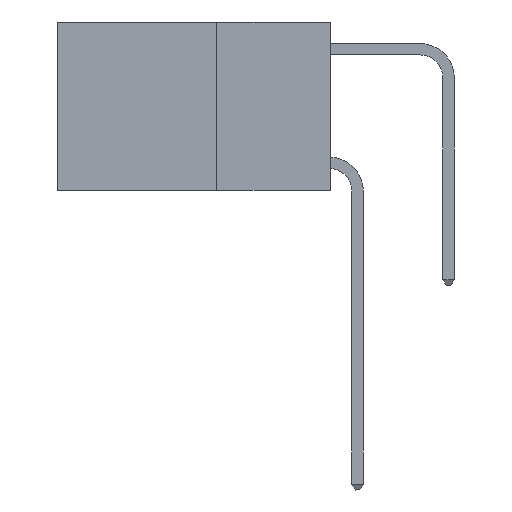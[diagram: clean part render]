
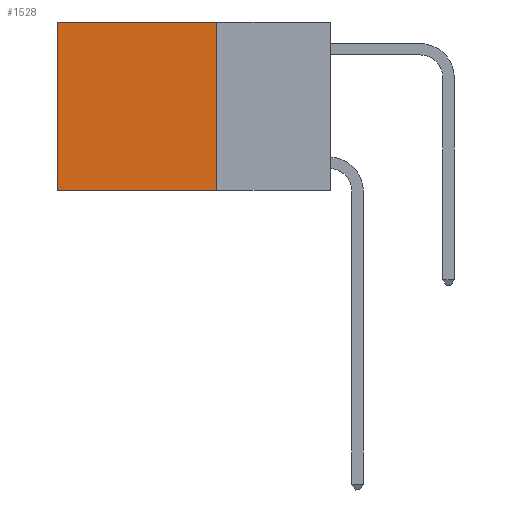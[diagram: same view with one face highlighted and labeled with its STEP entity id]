
A CAD part, left-side view. The second image highlights one B-rep face of the part: STEP entity #1528.
In plain terms, the highlighted planar face has unit normal (-1, 0, 0).
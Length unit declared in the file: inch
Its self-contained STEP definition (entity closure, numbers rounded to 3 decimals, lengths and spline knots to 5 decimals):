
#46 = ORIENTED_EDGE ( 'NONE', *, *, #2604, .T. ) ;
#294 = CARTESIAN_POINT ( 'NONE',  ( 0.2625, 0.6, 0. ) ) ;
#338 = CARTESIAN_POINT ( 'NONE',  ( 0.2625, 0.25, 0. ) ) ;
#368 = CARTESIAN_POINT ( 'NONE',  ( 0.2625, 0.25, -0.37 ) ) ;
#726 = ORIENTED_EDGE ( 'NONE', *, *, #10344, .F. ) ;
#1406 = LINE ( 'NONE', #1789, #10536 ) ;
#1528 = ADVANCED_FACE ( 'NONE', ( #6021 ), #5785, .F. ) ;
#1664 = CARTESIAN_POINT ( 'NONE',  ( 0.2625, 0.6, 0. ) ) ;
#1789 = CARTESIAN_POINT ( 'NONE',  ( 0.2625, 0.25, 0. ) ) ;
#2604 = EDGE_CURVE ( 'NONE', #6436, #3907, #1406, .T. ) ;
#2663 = EDGE_LOOP ( 'NONE', ( #2722, #10533, #726, #46 ) ) ;
#2722 = ORIENTED_EDGE ( 'NONE', *, *, #5236, .T. ) ;
#3270 = VECTOR ( 'NONE', #9887, 39.37008 ) ;
#3473 = AXIS2_PLACEMENT_3D ( 'NONE', #4329, #7424, #7288 ) ;
#3683 = VERTEX_POINT ( 'NONE', #368 ) ;
#3907 = VERTEX_POINT ( 'NONE', #1664 ) ;
#4329 = CARTESIAN_POINT ( 'NONE',  ( 0.2625, 0.25, 0. ) ) ;
#5236 = EDGE_CURVE ( 'NONE', #3907, #9741, #11048, .T. ) ;
#5620 = CARTESIAN_POINT ( 'NONE',  ( 0.2625, 0.25, 0. ) ) ;
#5785 = PLANE ( 'NONE',  #3473 ) ;
#5963 = VECTOR ( 'NONE', #11288, 39.37008 ) ;
#6021 = FACE_OUTER_BOUND ( 'NONE', #2663, .T. ) ;
#6254 = LINE ( 'NONE', #7150, #5963 ) ;
#6436 = VERTEX_POINT ( 'NONE', #338 ) ;
#7150 = CARTESIAN_POINT ( 'NONE',  ( 0.2625, 0.25, -0.37 ) ) ;
#7288 = DIRECTION ( 'NONE',  ( 0., 0., -1. ) ) ;
#7326 = EDGE_CURVE ( 'NONE', #3683, #9741, #6254, .T. ) ;
#7424 = DIRECTION ( 'NONE',  ( 1., 0., 0. ) ) ;
#7603 = DIRECTION ( 'NONE',  ( 0., 0., -1. ) ) ;
#7933 = LINE ( 'NONE', #5620, #3270 ) ;
#9741 = VERTEX_POINT ( 'NONE', #9936 ) ;
#9748 = DIRECTION ( 'NONE',  ( 0., 1., 0. ) ) ;
#9887 = DIRECTION ( 'NONE',  ( 0., 0., -1. ) ) ;
#9936 = CARTESIAN_POINT ( 'NONE',  ( 0.2625, 0.6, -0.37 ) ) ;
#10344 = EDGE_CURVE ( 'NONE', #6436, #3683, #7933, .T. ) ;
#10533 = ORIENTED_EDGE ( 'NONE', *, *, #7326, .F. ) ;
#10536 = VECTOR ( 'NONE', #9748, 39.37008 ) ;
#10813 = VECTOR ( 'NONE', #7603, 39.37008 ) ;
#11048 = LINE ( 'NONE', #294, #10813 ) ;
#11288 = DIRECTION ( 'NONE',  ( 0., 1., 0. ) ) ;
